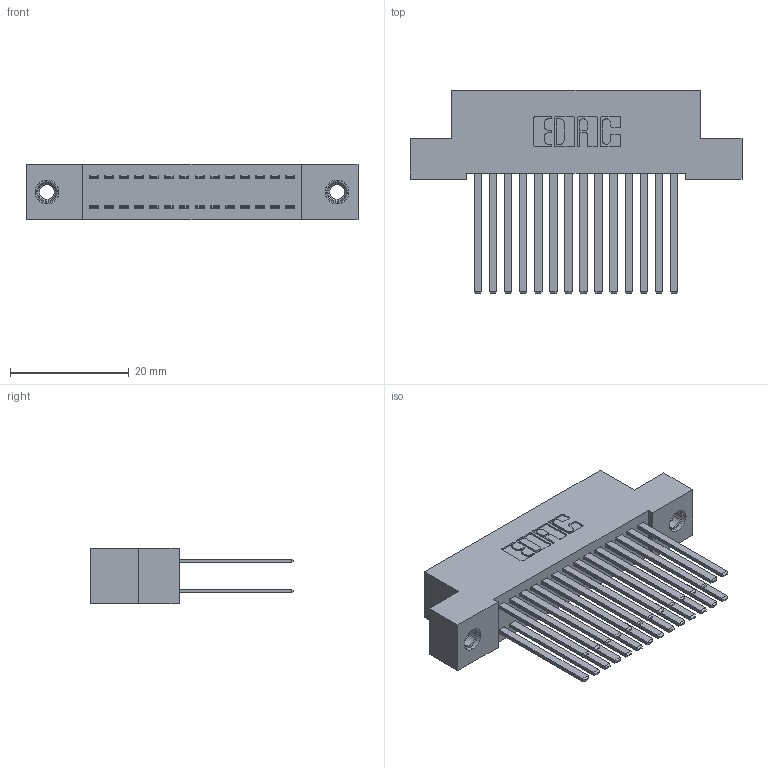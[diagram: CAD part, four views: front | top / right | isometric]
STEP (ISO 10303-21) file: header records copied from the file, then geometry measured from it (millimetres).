
FILE_DESCRIPTION (( 'STEP AP203' ), '1' );
FILE_NAME ('392-028-544-207.STEP', '2018-08-15T21:19:17', ( '' ), ( '' ), 'SwSTEP 2.0', 'SolidWorks 2016', '' );
FILE_SCHEMA (( 'CONFIG_CONTROL_DESIGN' ));
Length unit declared in the file: inch
Products named in the file (4): 345-292-001_345-293-144; 345-250-001_345-250-005-103; 392-028-544-207; 342 Part_TI
Assembly tree (31 placements, depth 2):
  392-028-544-207
    342 Part_TI
    345-292-001_345-293-144  x28
    345-250-001_345-250-005-103  x2
Bounding box: 55.88 x 34.3 x 9.4 mm (x, y, z)
Volume: 5268.1 mm3; surface area: 8998 mm2
Topology: 31 solids, 31 shells, 1458 faces, 4271 edges, 2802 vertices
Faces by surface type: plane 994, cylinder 448, cone 12, torus 4
Entity records: 13498 total; most frequent: CARTESIAN_POINT 2249, ORIENTED_EDGE 2178, DIRECTION 1999, EDGE_CURVE 1089, LINE 945, VECTOR 945, VERTEX_POINT 720, AXIS2_PLACEMENT_3D 527
